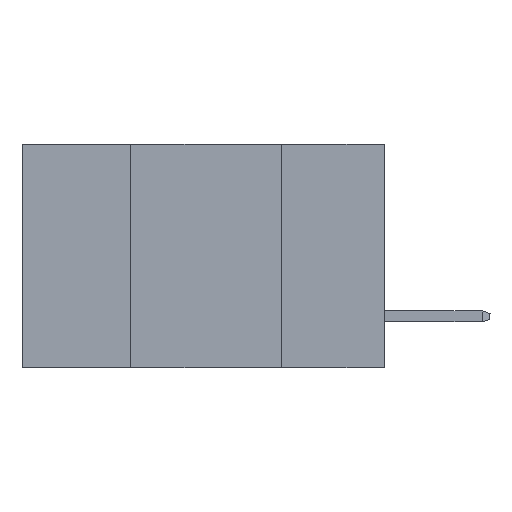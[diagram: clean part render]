
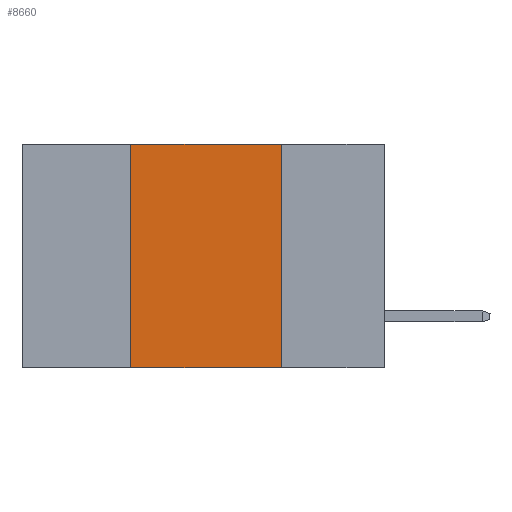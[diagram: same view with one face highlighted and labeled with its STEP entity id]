
A CAD part, left-side view. The second image highlights one B-rep face of the part: STEP entity #8660.
In plain terms, the highlighted planar face has unit normal (-1, 0, 0).
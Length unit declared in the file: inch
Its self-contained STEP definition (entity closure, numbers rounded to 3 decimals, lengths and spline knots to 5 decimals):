
#18 = EDGE_CURVE ( 'NONE', #3788, #9125, #582, .T. ) ;
#255 = VECTOR ( 'NONE', #6212, 39.37008 ) ;
#525 = EDGE_CURVE ( 'NONE', #9125, #7639, #5257, .T. ) ;
#559 = CARTESIAN_POINT ( 'NONE',  ( 0., 0.42, -0.37 ) ) ;
#582 = LINE ( 'NONE', #3002, #255 ) ;
#1315 = CARTESIAN_POINT ( 'NONE',  ( 0., 0.6, 0. ) ) ;
#1338 = CARTESIAN_POINT ( 'NONE',  ( 0., 0.6, 0. ) ) ;
#1589 = CARTESIAN_POINT ( 'NONE',  ( 0., 0.6, -0.37 ) ) ;
#2014 = DIRECTION ( 'NONE',  ( 0., 0., -1. ) ) ;
#2064 = CARTESIAN_POINT ( 'NONE',  ( 0., 0.17, -0.37 ) ) ;
#2479 = ORIENTED_EDGE ( 'NONE', *, *, #525, .F. ) ;
#2942 = DIRECTION ( 'NONE',  ( 0., -1., 0. ) ) ;
#3002 = CARTESIAN_POINT ( 'NONE',  ( 0., 0.42, -0.37 ) ) ;
#3234 = ORIENTED_EDGE ( 'NONE', *, *, #18, .F. ) ;
#3330 = EDGE_LOOP ( 'NONE', ( #10418, #2479, #3234, #10224 ) ) ;
#3531 = CARTESIAN_POINT ( 'NONE',  ( 0., 0.17, -0.37 ) ) ;
#3546 = FACE_OUTER_BOUND ( 'NONE', #3330, .T. ) ;
#3694 = DIRECTION ( 'NONE',  ( 0., 0., -1. ) ) ;
#3788 = VERTEX_POINT ( 'NONE', #559 ) ;
#3893 = CARTESIAN_POINT ( 'NONE',  ( 0., 0.17, 0. ) ) ;
#4075 = VECTOR ( 'NONE', #8809, 39.37008 ) ;
#4865 = VECTOR ( 'NONE', #3694, 39.37008 ) ;
#5177 = VERTEX_POINT ( 'NONE', #2064 ) ;
#5257 = LINE ( 'NONE', #1315, #10402 ) ;
#6212 = DIRECTION ( 'NONE',  ( 0., 0., 1. ) ) ;
#6298 = LINE ( 'NONE', #1589, #4075 ) ;
#6773 = LINE ( 'NONE', #3531, #4865 ) ;
#7223 = EDGE_CURVE ( 'NONE', #3788, #5177, #6298, .T. ) ;
#7639 = VERTEX_POINT ( 'NONE', #3893 ) ;
#7801 = PLANE ( 'NONE',  #8257 ) ;
#8257 = AXIS2_PLACEMENT_3D ( 'NONE', #1338, #10036, #2014 ) ;
#8660 = ADVANCED_FACE ( 'NONE', ( #3546 ), #7801, .F. ) ;
#8809 = DIRECTION ( 'NONE',  ( 0., -1., 0. ) ) ;
#9089 = EDGE_CURVE ( 'NONE', #7639, #5177, #6773, .T. ) ;
#9125 = VERTEX_POINT ( 'NONE', #9220 ) ;
#9220 = CARTESIAN_POINT ( 'NONE',  ( 0., 0.42, 0. ) ) ;
#10036 = DIRECTION ( 'NONE',  ( 1., 0., 0. ) ) ;
#10224 = ORIENTED_EDGE ( 'NONE', *, *, #7223, .T. ) ;
#10402 = VECTOR ( 'NONE', #2942, 39.37008 ) ;
#10418 = ORIENTED_EDGE ( 'NONE', *, *, #9089, .F. ) ;
